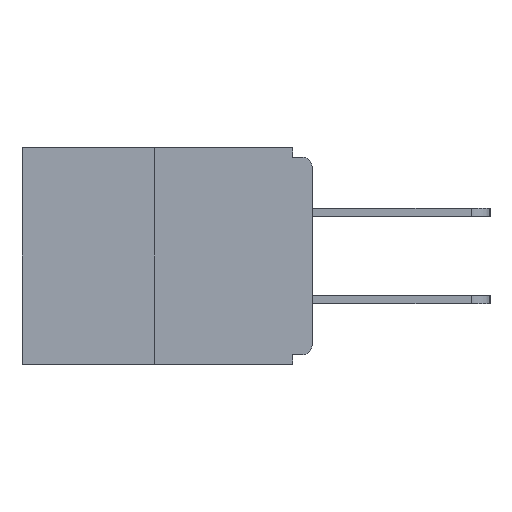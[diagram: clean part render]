
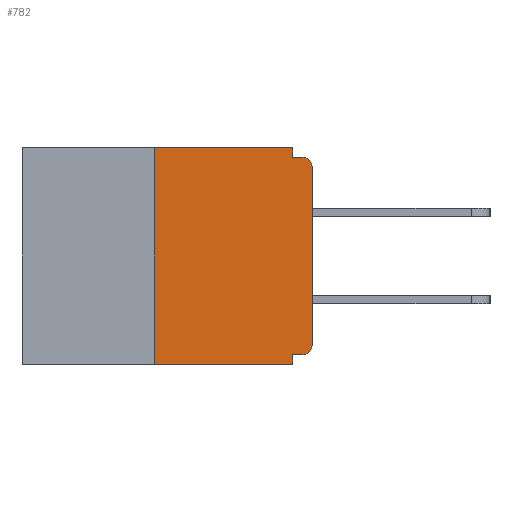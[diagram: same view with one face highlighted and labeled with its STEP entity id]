
A CAD part, left-side view. The second image highlights one B-rep face of the part: STEP entity #782.
In plain terms, the highlighted planar face has unit normal (-1, 0, 0).
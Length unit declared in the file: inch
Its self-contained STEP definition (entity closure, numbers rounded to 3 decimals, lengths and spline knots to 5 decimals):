
#102 = EDGE_CURVE ( 'NONE', #28239, #7408, #2558, .T. ) ;
#237 = CARTESIAN_POINT ( 'NONE',  ( 0., 0.25, 0. ) ) ;
#714 = AXIS2_PLACEMENT_3D ( 'NONE', #22426, #7369, #22604 ) ;
#782 = ADVANCED_FACE ( 'NONE', ( #8442 ), #18332, .F. ) ;
#848 = CARTESIAN_POINT ( 'NONE',  ( 0., 0., -0.015 ) ) ;
#865 = CARTESIAN_POINT ( 'NONE',  ( 0., 0.015, -0.03 ) ) ;
#903 = LINE ( 'NONE', #27433, #17857 ) ;
#975 = DIRECTION ( 'NONE',  ( 0., 0., -1. ) ) ;
#1441 = EDGE_CURVE ( 'NONE', #5817, #28239, #8020, .T. ) ;
#2208 = CARTESIAN_POINT ( 'NONE',  ( 0., 0.015, -0.328 ) ) ;
#2354 = EDGE_CURVE ( 'NONE', #18739, #8224, #21397, .T. ) ;
#2558 = LINE ( 'NONE', #848, #14322 ) ;
#3419 = LINE ( 'NONE', #237, #13147 ) ;
#3632 = CARTESIAN_POINT ( 'NONE',  ( 0., 0.25, -0.343 ) ) ;
#4080 = CARTESIAN_POINT ( 'NONE',  ( 0., 0.46, 0. ) ) ;
#4084 = CARTESIAN_POINT ( 'NONE',  ( 0., 0.015, -0.313 ) ) ;
#4631 = CARTESIAN_POINT ( 'NONE',  ( 0., 0., 0. ) ) ;
#4689 = DIRECTION ( 'NONE',  ( 0., 0., 1. ) ) ;
#4705 = CARTESIAN_POINT ( 'NONE',  ( 0., 0.031, -0.343 ) ) ;
#4985 = AXIS2_PLACEMENT_3D ( 'NONE', #4084, #10698, #19543 ) ;
#5154 = CARTESIAN_POINT ( 'NONE',  ( 0., 0., -0.313 ) ) ;
#5399 = VERTEX_POINT ( 'NONE', #3632 ) ;
#5765 = CARTESIAN_POINT ( 'NONE',  ( 0., 0.46, -0.343 ) ) ;
#5817 = VERTEX_POINT ( 'NONE', #25926 ) ;
#6274 = ORIENTED_EDGE ( 'NONE', *, *, #23680, .F. ) ;
#6394 = CIRCLE ( 'NONE', #19664, 0.015 ) ;
#6656 = LINE ( 'NONE', #20319, #12513 ) ;
#6817 = CARTESIAN_POINT ( 'NONE',  ( 0., 0.031, -0.015 ) ) ;
#7069 = DIRECTION ( 'NONE',  ( 0., 1., 0. ) ) ;
#7181 = EDGE_CURVE ( 'NONE', #5399, #18658, #3419, .T. ) ;
#7369 = DIRECTION ( 'NONE',  ( 1., 0., 0. ) ) ;
#7408 = VERTEX_POINT ( 'NONE', #16470 ) ;
#8020 = LINE ( 'NONE', #27654, #24922 ) ;
#8224 = VERTEX_POINT ( 'NONE', #5154 ) ;
#8442 = FACE_OUTER_BOUND ( 'NONE', #12432, .T. ) ;
#9725 = VECTOR ( 'NONE', #24533, 39.37008 ) ;
#10698 = DIRECTION ( 'NONE',  ( -1., 0., 0. ) ) ;
#12134 = VERTEX_POINT ( 'NONE', #13197 ) ;
#12345 = DIRECTION ( 'NONE',  ( 0., 0., -1. ) ) ;
#12432 = EDGE_LOOP ( 'NONE', ( #6274, #25407, #26312, #27611, #13143, #23028, #22329, #16469, #17536, #24417 ) ) ;
#12513 = VECTOR ( 'NONE', #7069, 39.37008 ) ;
#12793 = LINE ( 'NONE', #4631, #9725 ) ;
#13143 = ORIENTED_EDGE ( 'NONE', *, *, #14106, .F. ) ;
#13147 = VECTOR ( 'NONE', #4689, 39.37008 ) ;
#13190 = DIRECTION ( 'NONE',  ( 0., -1., 0. ) ) ;
#13197 = CARTESIAN_POINT ( 'NONE',  ( 0., 0., -0.03 ) ) ;
#14106 = EDGE_CURVE ( 'NONE', #18739, #20749, #6656, .T. ) ;
#14322 = VECTOR ( 'NONE', #25288, 39.37008 ) ;
#16469 = ORIENTED_EDGE ( 'NONE', *, *, #18305, .T. ) ;
#16470 = CARTESIAN_POINT ( 'NONE',  ( 0., 0.015, -0.015 ) ) ;
#17442 = VECTOR ( 'NONE', #13190, 39.37008 ) ;
#17536 = ORIENTED_EDGE ( 'NONE', *, *, #102, .F. ) ;
#17857 = VECTOR ( 'NONE', #975, 39.37008 ) ;
#18305 = EDGE_CURVE ( 'NONE', #12134, #7408, #6394, .T. ) ;
#18332 = PLANE ( 'NONE',  #714 ) ;
#18455 = DIRECTION ( 'NONE',  ( 0., 0., -1. ) ) ;
#18658 = VERTEX_POINT ( 'NONE', #21662 ) ;
#18739 = VERTEX_POINT ( 'NONE', #2208 ) ;
#19465 = VECTOR ( 'NONE', #27667, 39.37008 ) ;
#19543 = DIRECTION ( 'NONE',  ( 0., 0., -1. ) ) ;
#19664 = AXIS2_PLACEMENT_3D ( 'NONE', #865, #23096, #18455 ) ;
#20319 = CARTESIAN_POINT ( 'NONE',  ( 0., 0., -0.328 ) ) ;
#20749 = VERTEX_POINT ( 'NONE', #24515 ) ;
#21397 = CIRCLE ( 'NONE', #4985, 0.015 ) ;
#21662 = CARTESIAN_POINT ( 'NONE',  ( 0., 0.25, 0. ) ) ;
#22196 = VERTEX_POINT ( 'NONE', #4705 ) ;
#22329 = ORIENTED_EDGE ( 'NONE', *, *, #25089, .T. ) ;
#22426 = CARTESIAN_POINT ( 'NONE',  ( 0., 0.46, 0. ) ) ;
#22598 = EDGE_CURVE ( 'NONE', #20749, #22196, #903, .T. ) ;
#22604 = DIRECTION ( 'NONE',  ( 0., 0., -1. ) ) ;
#23028 = ORIENTED_EDGE ( 'NONE', *, *, #2354, .T. ) ;
#23096 = DIRECTION ( 'NONE',  ( -1., 0., 0. ) ) ;
#23336 = LINE ( 'NONE', #4080, #17442 ) ;
#23680 = EDGE_CURVE ( 'NONE', #18658, #5817, #23336, .T. ) ;
#24417 = ORIENTED_EDGE ( 'NONE', *, *, #1441, .F. ) ;
#24515 = CARTESIAN_POINT ( 'NONE',  ( 0., 0.031, -0.328 ) ) ;
#24533 = DIRECTION ( 'NONE',  ( 0., 0., 1. ) ) ;
#24805 = EDGE_CURVE ( 'NONE', #5399, #22196, #28103, .T. ) ;
#24922 = VECTOR ( 'NONE', #12345, 39.37008 ) ;
#25089 = EDGE_CURVE ( 'NONE', #8224, #12134, #12793, .T. ) ;
#25288 = DIRECTION ( 'NONE',  ( 0., -1., 0. ) ) ;
#25407 = ORIENTED_EDGE ( 'NONE', *, *, #7181, .F. ) ;
#25926 = CARTESIAN_POINT ( 'NONE',  ( 0., 0.031, 0. ) ) ;
#26312 = ORIENTED_EDGE ( 'NONE', *, *, #24805, .T. ) ;
#27433 = CARTESIAN_POINT ( 'NONE',  ( 0., 0.031, -0.343 ) ) ;
#27611 = ORIENTED_EDGE ( 'NONE', *, *, #22598, .F. ) ;
#27654 = CARTESIAN_POINT ( 'NONE',  ( 0., 0.031, 0. ) ) ;
#27667 = DIRECTION ( 'NONE',  ( 0., -1., 0. ) ) ;
#28103 = LINE ( 'NONE', #5765, #19465 ) ;
#28239 = VERTEX_POINT ( 'NONE', #6817 ) ;
